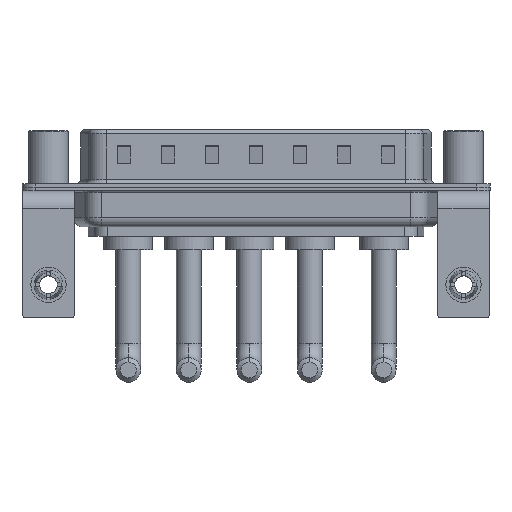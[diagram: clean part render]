
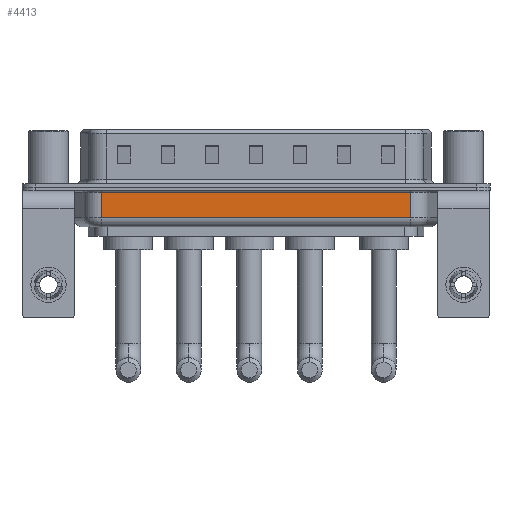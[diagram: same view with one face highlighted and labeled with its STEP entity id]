
A CAD part, front view. The second image highlights one B-rep face of the part: STEP entity #4413.
In plain terms, the highlighted planar face has unit normal (0, -1, 0).
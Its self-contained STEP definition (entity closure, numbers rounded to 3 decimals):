
#1039 = DIRECTION ( 'NONE',  ( 0., 0., 1. ) ) ;
#2128 = VECTOR ( 'NONE', #9368, 1000. ) ;
#3747 = LINE ( 'NONE', #12564, #6156 ) ;
#4074 = EDGE_CURVE ( 'NONE', #12667, #15165, #3747, .T. ) ;
#4099 = CARTESIAN_POINT ( 'NONE',  ( 6.006, -5.35, -0.65 ) ) ;
#4257 = ORIENTED_EDGE ( 'NONE', *, *, #9284, .T. ) ;
#4413 = ADVANCED_FACE ( 'NONE', ( #16366 ), #5219, .F. ) ;
#4478 = AXIS2_PLACEMENT_3D ( 'NONE', #4591, #7411, #12341 ) ;
#4591 = CARTESIAN_POINT ( 'NONE',  ( 6.006, -5.35, -4.5 ) ) ;
#5219 = PLANE ( 'NONE',  #4478 ) ;
#6096 = LINE ( 'NONE', #9001, #2128 ) ;
#6156 = VECTOR ( 'NONE', #1039, 1000. ) ;
#6333 = CARTESIAN_POINT ( 'NONE',  ( 41.044, -5.35, -3.5 ) ) ;
#7102 = CARTESIAN_POINT ( 'NONE',  ( 6.006, -5.35, -0.65 ) ) ;
#7156 = CARTESIAN_POINT ( 'NONE',  ( 6.006, -5.35, -3.5 ) ) ;
#7316 = VECTOR ( 'NONE', #11403, 1000. ) ;
#7411 = DIRECTION ( 'NONE',  ( 0., 1., 0. ) ) ;
#7617 = EDGE_CURVE ( 'NONE', #14898, #15165, #14214, .T. ) ;
#8996 = VERTEX_POINT ( 'NONE', #6333 ) ;
#9001 = CARTESIAN_POINT ( 'NONE',  ( 41.044, -5.35, -4.5 ) ) ;
#9284 = EDGE_CURVE ( 'NONE', #12667, #8996, #11711, .T. ) ;
#9368 = DIRECTION ( 'NONE',  ( 0., 0., 1. ) ) ;
#9620 = ORIENTED_EDGE ( 'NONE', *, *, #15067, .T. ) ;
#10106 = EDGE_LOOP ( 'NONE', ( #10352, #4257, #9620, #11985 ) ) ;
#10352 = ORIENTED_EDGE ( 'NONE', *, *, #4074, .F. ) ;
#11340 = CARTESIAN_POINT ( 'NONE',  ( 41.044, -5.35, -0.65 ) ) ;
#11403 = DIRECTION ( 'NONE',  ( -1., 0., 0. ) ) ;
#11711 = LINE ( 'NONE', #7156, #12545 ) ;
#11849 = CARTESIAN_POINT ( 'NONE',  ( 6.006, -5.35, -3.5 ) ) ;
#11985 = ORIENTED_EDGE ( 'NONE', *, *, #7617, .T. ) ;
#12341 = DIRECTION ( 'NONE',  ( 0., 0., 1. ) ) ;
#12545 = VECTOR ( 'NONE', #18204, 1000. ) ;
#12564 = CARTESIAN_POINT ( 'NONE',  ( 6.006, -5.35, -4.5 ) ) ;
#12667 = VERTEX_POINT ( 'NONE', #11849 ) ;
#14214 = LINE ( 'NONE', #7102, #7316 ) ;
#14898 = VERTEX_POINT ( 'NONE', #11340 ) ;
#15067 = EDGE_CURVE ( 'NONE', #8996, #14898, #6096, .T. ) ;
#15165 = VERTEX_POINT ( 'NONE', #4099 ) ;
#16366 = FACE_OUTER_BOUND ( 'NONE', #10106, .T. ) ;
#18204 = DIRECTION ( 'NONE',  ( 1., 0., 0. ) ) ;
